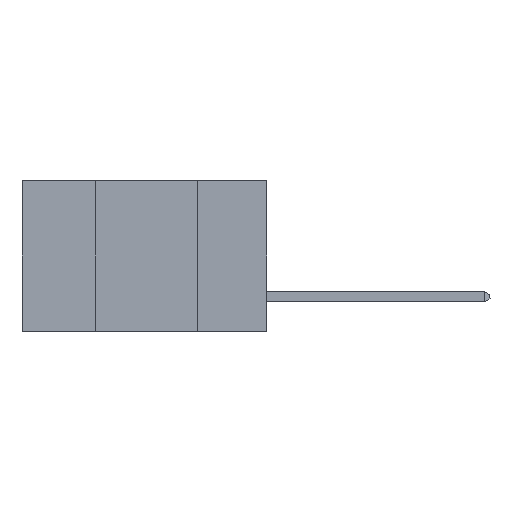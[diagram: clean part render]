
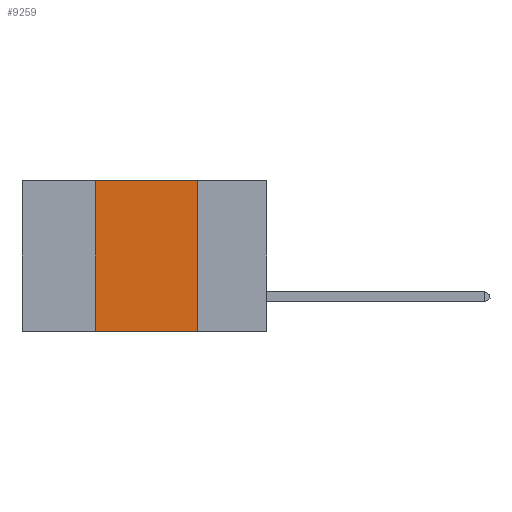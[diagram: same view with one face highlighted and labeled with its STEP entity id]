
A CAD part, left-side view. The second image highlights one B-rep face of the part: STEP entity #9259.
In plain terms, the highlighted planar face has unit normal (-1, 0, 0).
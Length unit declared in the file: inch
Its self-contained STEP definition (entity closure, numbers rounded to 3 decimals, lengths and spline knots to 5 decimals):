
#197 = VECTOR ( 'NONE', #11677, 39.37008 ) ;
#460 = ORIENTED_EDGE ( 'NONE', *, *, #10951, .F. ) ;
#2199 = CARTESIAN_POINT ( 'NONE',  ( 0., 0.42, 0. ) ) ;
#3022 = CARTESIAN_POINT ( 'NONE',  ( 0., 0.6, -0.37 ) ) ;
#3716 = EDGE_CURVE ( 'NONE', #10210, #5072, #8329, .T. ) ;
#4144 = VECTOR ( 'NONE', #8032, 39.37008 ) ;
#4659 = ORIENTED_EDGE ( 'NONE', *, *, #6086, .T. ) ;
#4803 = CARTESIAN_POINT ( 'NONE',  ( 0., 0.6, 0. ) ) ;
#5072 = VERTEX_POINT ( 'NONE', #11198 ) ;
#5292 = FACE_OUTER_BOUND ( 'NONE', #7146, .T. ) ;
#5665 = VERTEX_POINT ( 'NONE', #10747 ) ;
#5911 = VECTOR ( 'NONE', #6577, 39.37008 ) ;
#6086 = EDGE_CURVE ( 'NONE', #5665, #12337, #8017, .T. ) ;
#6577 = DIRECTION ( 'NONE',  ( 0., -1., 0. ) ) ;
#6625 = CARTESIAN_POINT ( 'NONE',  ( 0., 0.17, 0. ) ) ;
#6744 = DIRECTION ( 'NONE',  ( 0., 0., -1. ) ) ;
#7146 = EDGE_LOOP ( 'NONE', ( #11705, #8011, #460, #4659 ) ) ;
#7495 = DIRECTION ( 'NONE',  ( 0., 0., -1. ) ) ;
#8011 = ORIENTED_EDGE ( 'NONE', *, *, #3716, .F. ) ;
#8017 = LINE ( 'NONE', #3022, #5911 ) ;
#8032 = DIRECTION ( 'NONE',  ( 0., 0., 1. ) ) ;
#8084 = CARTESIAN_POINT ( 'NONE',  ( 0., 0.17, -0.37 ) ) ;
#8329 = LINE ( 'NONE', #11440, #197 ) ;
#8334 = VECTOR ( 'NONE', #7495, 39.37008 ) ;
#9184 = EDGE_CURVE ( 'NONE', #5072, #12337, #11347, .T. ) ;
#9259 = ADVANCED_FACE ( 'NONE', ( #5292 ), #11270, .F. ) ;
#10210 = VERTEX_POINT ( 'NONE', #12051 ) ;
#10292 = AXIS2_PLACEMENT_3D ( 'NONE', #4803, #12154, #6744 ) ;
#10747 = CARTESIAN_POINT ( 'NONE',  ( 0., 0.42, -0.37 ) ) ;
#10951 = EDGE_CURVE ( 'NONE', #5665, #10210, #11576, .T. ) ;
#11198 = CARTESIAN_POINT ( 'NONE',  ( 0., 0.17, 0. ) ) ;
#11270 = PLANE ( 'NONE',  #10292 ) ;
#11347 = LINE ( 'NONE', #6625, #8334 ) ;
#11440 = CARTESIAN_POINT ( 'NONE',  ( 0., 0.6, 0. ) ) ;
#11576 = LINE ( 'NONE', #2199, #4144 ) ;
#11677 = DIRECTION ( 'NONE',  ( 0., -1., 0. ) ) ;
#11705 = ORIENTED_EDGE ( 'NONE', *, *, #9184, .F. ) ;
#12051 = CARTESIAN_POINT ( 'NONE',  ( 0., 0.42, 0. ) ) ;
#12154 = DIRECTION ( 'NONE',  ( 1., 0., 0. ) ) ;
#12337 = VERTEX_POINT ( 'NONE', #8084 ) ;
